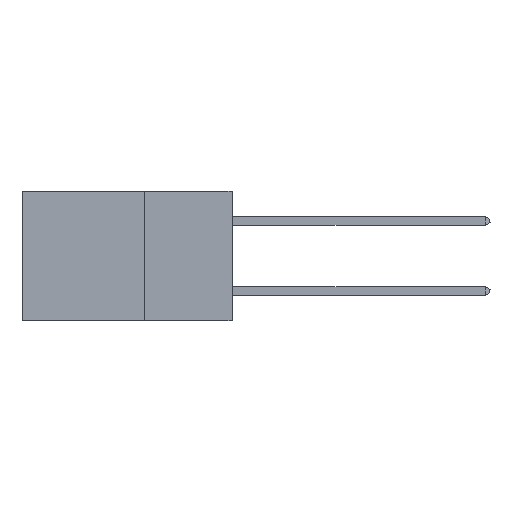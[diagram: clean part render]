
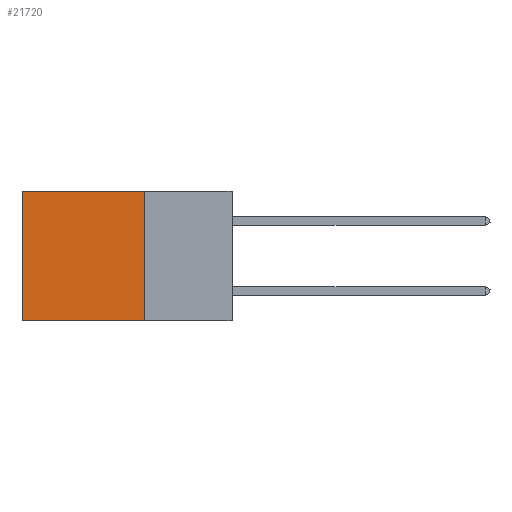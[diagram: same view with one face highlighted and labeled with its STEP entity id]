
A CAD part, left-side view. The second image highlights one B-rep face of the part: STEP entity #21720.
In plain terms, the highlighted planar face has unit normal (-1, 0, 0).
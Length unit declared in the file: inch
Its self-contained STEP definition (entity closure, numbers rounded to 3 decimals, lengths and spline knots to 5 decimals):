
#1179 = DIRECTION ( 'NONE',  ( 0., 0., -1. ) ) ;
#2531 = AXIS2_PLACEMENT_3D ( 'NONE', #38892, #32933, #14283 ) ;
#2631 = VECTOR ( 'NONE', #6063, 39.37008 ) ;
#2714 = DIRECTION ( 'NONE',  ( 0., 1., 0. ) ) ;
#3345 = EDGE_CURVE ( 'NONE', #9824, #37771, #11110, .T. ) ;
#4614 = VECTOR ( 'NONE', #33833, 39.37008 ) ;
#6063 = DIRECTION ( 'NONE',  ( 0., 1., 0. ) ) ;
#7176 = LINE ( 'NONE', #18572, #38377 ) ;
#7690 = CARTESIAN_POINT ( 'NONE',  ( 0.2875, 0.25, 0. ) ) ;
#8827 = CARTESIAN_POINT ( 'NONE',  ( 0.2875, 0.25, 0. ) ) ;
#9824 = VERTEX_POINT ( 'NONE', #7690 ) ;
#10444 = ORIENTED_EDGE ( 'NONE', *, *, #25050, .T. ) ;
#11110 = LINE ( 'NONE', #37148, #2631 ) ;
#11183 = CARTESIAN_POINT ( 'NONE',  ( 0.2875, 0.25, -0.37 ) ) ;
#13082 = LINE ( 'NONE', #8827, #4614 ) ;
#13829 = VERTEX_POINT ( 'NONE', #27583 ) ;
#14283 = DIRECTION ( 'NONE',  ( 0., 0., -1. ) ) ;
#14386 = ORIENTED_EDGE ( 'NONE', *, *, #3345, .T. ) ;
#17311 = PLANE ( 'NONE',  #2531 ) ;
#18572 = CARTESIAN_POINT ( 'NONE',  ( 0.2875, 0.25, -0.37 ) ) ;
#19597 = EDGE_CURVE ( 'NONE', #25802, #13829, #7176, .T. ) ;
#21720 = ADVANCED_FACE ( 'NONE', ( #27699 ), #17311, .F. ) ;
#23540 = VECTOR ( 'NONE', #1179, 39.37008 ) ;
#25050 = EDGE_CURVE ( 'NONE', #37771, #13829, #31716, .T. ) ;
#25802 = VERTEX_POINT ( 'NONE', #11183 ) ;
#25976 = EDGE_CURVE ( 'NONE', #9824, #25802, #13082, .T. ) ;
#26235 = ORIENTED_EDGE ( 'NONE', *, *, #25976, .F. ) ;
#27583 = CARTESIAN_POINT ( 'NONE',  ( 0.2875, 0.6, -0.37 ) ) ;
#27699 = FACE_OUTER_BOUND ( 'NONE', #33626, .T. ) ;
#31350 = ORIENTED_EDGE ( 'NONE', *, *, #19597, .F. ) ;
#31716 = LINE ( 'NONE', #35475, #23540 ) ;
#32029 = CARTESIAN_POINT ( 'NONE',  ( 0.2875, 0.6, 0. ) ) ;
#32933 = DIRECTION ( 'NONE',  ( 1., 0., 0. ) ) ;
#33626 = EDGE_LOOP ( 'NONE', ( #10444, #31350, #26235, #14386 ) ) ;
#33833 = DIRECTION ( 'NONE',  ( 0., 0., -1. ) ) ;
#35475 = CARTESIAN_POINT ( 'NONE',  ( 0.2875, 0.6, 0. ) ) ;
#37148 = CARTESIAN_POINT ( 'NONE',  ( 0.2875, 0.25, 0. ) ) ;
#37771 = VERTEX_POINT ( 'NONE', #32029 ) ;
#38377 = VECTOR ( 'NONE', #2714, 39.37008 ) ;
#38892 = CARTESIAN_POINT ( 'NONE',  ( 0.2875, 0.25, 0. ) ) ;
